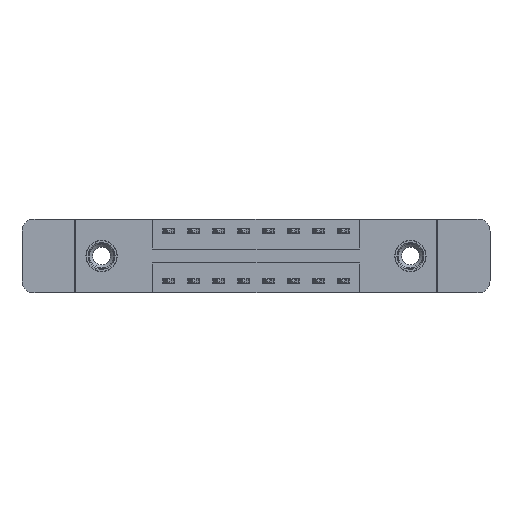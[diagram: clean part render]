
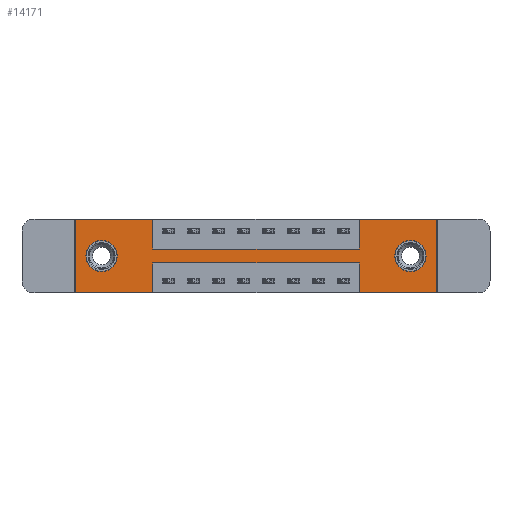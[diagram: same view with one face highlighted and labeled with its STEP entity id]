
A CAD part, front view. The second image highlights one B-rep face of the part: STEP entity #14171.
In plain terms, the highlighted planar face has unit normal (0, -1, 0).
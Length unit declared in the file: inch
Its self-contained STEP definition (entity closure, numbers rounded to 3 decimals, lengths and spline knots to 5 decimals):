
#9 = CARTESIAN_POINT ( 'NONE',  ( 1.6775, 0., -0.185 ) ) ;
#105 = ORIENTED_EDGE ( 'NONE', *, *, #8031, .F. ) ;
#212 = VECTOR ( 'NONE', #14831, 39.37008 ) ;
#493 = VERTEX_POINT ( 'NONE', #2565 ) ;
#850 = CIRCLE ( 'NONE', #13565, 0.078 ) ;
#884 = CARTESIAN_POINT ( 'NONE',  ( 0., 0., -0.37 ) ) ;
#892 = DIRECTION ( 'NONE',  ( 0., 0., -1. ) ) ;
#1053 = DIRECTION ( 'NONE',  ( 0., 0., -1. ) ) ;
#1204 = LINE ( 'NONE', #8077, #2448 ) ;
#1249 = VERTEX_POINT ( 'NONE', #8143 ) ;
#1659 = CIRCLE ( 'NONE', #5399, 0.078 ) ;
#1745 = CARTESIAN_POINT ( 'NONE',  ( 1.6775, 0., -0.185 ) ) ;
#1794 = DIRECTION ( 'NONE',  ( 0., 0., 1. ) ) ;
#1838 = EDGE_CURVE ( 'NONE', #9405, #1249, #10299, .T. ) ;
#1860 = DIRECTION ( 'NONE',  ( 0., 1., 0. ) ) ;
#1910 = DIRECTION ( 'NONE',  ( 0., 0., -1. ) ) ;
#1924 = CARTESIAN_POINT ( 'NONE',  ( 0., 0., -0.37 ) ) ;
#2002 = EDGE_CURVE ( 'NONE', #15263, #4245, #850, .T. ) ;
#2095 = CARTESIAN_POINT ( 'NONE',  ( 0.3875, 0., -0.22 ) ) ;
#2115 = EDGE_CURVE ( 'NONE', #8265, #6887, #10602, .T. ) ;
#2167 = EDGE_CURVE ( 'NONE', #6887, #2943, #5915, .T. ) ;
#2219 = EDGE_CURVE ( 'NONE', #12027, #9405, #13260, .T. ) ;
#2325 = ORIENTED_EDGE ( 'NONE', *, *, #8556, .F. ) ;
#2326 = DIRECTION ( 'NONE',  ( 0., 0., -1. ) ) ;
#2348 = ORIENTED_EDGE ( 'NONE', *, *, #10977, .F. ) ;
#2448 = VECTOR ( 'NONE', #13074, 39.37008 ) ;
#2565 = CARTESIAN_POINT ( 'NONE',  ( 1.81, 0., 0. ) ) ;
#2687 = LINE ( 'NONE', #14337, #8946 ) ;
#2885 = EDGE_LOOP ( 'NONE', ( #11225, #3592 ) ) ;
#2943 = VERTEX_POINT ( 'NONE', #4405 ) ;
#3103 = CARTESIAN_POINT ( 'NONE',  ( 1.4225, 0., 0. ) ) ;
#3215 = ORIENTED_EDGE ( 'NONE', *, *, #14825, .F. ) ;
#3223 = PLANE ( 'NONE',  #6197 ) ;
#3311 = VECTOR ( 'NONE', #1794, 39.37008 ) ;
#3425 = ORIENTED_EDGE ( 'NONE', *, *, #1838, .F. ) ;
#3592 = ORIENTED_EDGE ( 'NONE', *, *, #7766, .T. ) ;
#3636 = DIRECTION ( 'NONE',  ( 0., 0., 1. ) ) ;
#3756 = VERTEX_POINT ( 'NONE', #4872 ) ;
#3757 = ORIENTED_EDGE ( 'NONE', *, *, #9633, .F. ) ;
#3869 = CARTESIAN_POINT ( 'NONE',  ( 0.3875, 0., 0. ) ) ;
#4245 = VERTEX_POINT ( 'NONE', #10963 ) ;
#4341 = CARTESIAN_POINT ( 'NONE',  ( 0.3875, 0., -0.15 ) ) ;
#4405 = CARTESIAN_POINT ( 'NONE',  ( 0.3875, 0., -0.22 ) ) ;
#4727 = DIRECTION ( 'NONE',  ( 1., 0., 0. ) ) ;
#4756 = DIRECTION ( 'NONE',  ( 0., 1., 0. ) ) ;
#4807 = VECTOR ( 'NONE', #13497, 39.37008 ) ;
#4872 = CARTESIAN_POINT ( 'NONE',  ( 1.81, 0., -0.37 ) ) ;
#4967 = CARTESIAN_POINT ( 'NONE',  ( 0.1325, 0., -0.185 ) ) ;
#5260 = DIRECTION ( 'NONE',  ( 0., 0., -1. ) ) ;
#5300 = LINE ( 'NONE', #10060, #212 ) ;
#5338 = CARTESIAN_POINT ( 'NONE',  ( 0., 0., -0.37 ) ) ;
#5340 = VECTOR ( 'NONE', #3636, 39.37008 ) ;
#5399 = AXIS2_PLACEMENT_3D ( 'NONE', #4967, #12008, #7393 ) ;
#5503 = ORIENTED_EDGE ( 'NONE', *, *, #10831, .F. ) ;
#5666 = LINE ( 'NONE', #12925, #8121 ) ;
#5884 = AXIS2_PLACEMENT_3D ( 'NONE', #1745, #13371, #5260 ) ;
#5915 = LINE ( 'NONE', #2095, #7087 ) ;
#6039 = EDGE_CURVE ( 'NONE', #8719, #9441, #14628, .T. ) ;
#6043 = CARTESIAN_POINT ( 'NONE',  ( 1.6775, 0., -0.263 ) ) ;
#6099 = EDGE_LOOP ( 'NONE', ( #9477, #8108 ) ) ;
#6107 = ORIENTED_EDGE ( 'NONE', *, *, #2167, .F. ) ;
#6197 = AXIS2_PLACEMENT_3D ( 'NONE', #8146, #6667, #892 ) ;
#6465 = DIRECTION ( 'NONE',  ( -1., 0., 0. ) ) ;
#6659 = CARTESIAN_POINT ( 'NONE',  ( 1.6775, 0., -0.107 ) ) ;
#6667 = DIRECTION ( 'NONE',  ( 0., -1., 0. ) ) ;
#6802 = VERTEX_POINT ( 'NONE', #3869 ) ;
#6887 = VERTEX_POINT ( 'NONE', #10922 ) ;
#7087 = VECTOR ( 'NONE', #9290, 39.37008 ) ;
#7271 = CARTESIAN_POINT ( 'NONE',  ( 0., 0., 0. ) ) ;
#7393 = DIRECTION ( 'NONE',  ( 0., 0., 1. ) ) ;
#7656 = VERTEX_POINT ( 'NONE', #9230 ) ;
#7681 = ORIENTED_EDGE ( 'NONE', *, *, #13968, .F. ) ;
#7714 = VECTOR ( 'NONE', #6465, 39.37008 ) ;
#7766 = EDGE_CURVE ( 'NONE', #9441, #8719, #8418, .T. ) ;
#7866 = VECTOR ( 'NONE', #1910, 39.37008 ) ;
#8031 = EDGE_CURVE ( 'NONE', #6802, #12027, #5300, .T. ) ;
#8077 = CARTESIAN_POINT ( 'NONE',  ( 0., 0., 0. ) ) ;
#8108 = ORIENTED_EDGE ( 'NONE', *, *, #2002, .T. ) ;
#8121 = VECTOR ( 'NONE', #1053, 39.37008 ) ;
#8143 = CARTESIAN_POINT ( 'NONE',  ( 1.4225, 0., 0. ) ) ;
#8146 = CARTESIAN_POINT ( 'NONE',  ( 0., 0., -0.37 ) ) ;
#8265 = VERTEX_POINT ( 'NONE', #13025 ) ;
#8413 = CARTESIAN_POINT ( 'NONE',  ( 0.3875, 0., -0.15 ) ) ;
#8418 = CIRCLE ( 'NONE', #10175, 0.078 ) ;
#8556 = EDGE_CURVE ( 'NONE', #8740, #7656, #1204, .T. ) ;
#8719 = VERTEX_POINT ( 'NONE', #6659 ) ;
#8740 = VERTEX_POINT ( 'NONE', #5338 ) ;
#8749 = LINE ( 'NONE', #7271, #13620 ) ;
#8881 = LINE ( 'NONE', #1924, #7714 ) ;
#8946 = VECTOR ( 'NONE', #4727, 39.37008 ) ;
#9100 = CARTESIAN_POINT ( 'NONE',  ( 0.3875, 0., -0.37 ) ) ;
#9230 = CARTESIAN_POINT ( 'NONE',  ( 0., 0., 0. ) ) ;
#9290 = DIRECTION ( 'NONE',  ( -1., 0., 0. ) ) ;
#9405 = VERTEX_POINT ( 'NONE', #14403 ) ;
#9441 = VERTEX_POINT ( 'NONE', #6043 ) ;
#9477 = ORIENTED_EDGE ( 'NONE', *, *, #11855, .T. ) ;
#9571 = CARTESIAN_POINT ( 'NONE',  ( 0.1325, 0., -0.263 ) ) ;
#9633 = EDGE_CURVE ( 'NONE', #3756, #8265, #11514, .T. ) ;
#9936 = ORIENTED_EDGE ( 'NONE', *, *, #11493, .F. ) ;
#10060 = CARTESIAN_POINT ( 'NONE',  ( 0.3875, 0., 0. ) ) ;
#10072 = CARTESIAN_POINT ( 'NONE',  ( 0.1325, 0., -0.185 ) ) ;
#10175 = AXIS2_PLACEMENT_3D ( 'NONE', #9, #4756, #2326 ) ;
#10229 = DIRECTION ( 'NONE',  ( 0., 0., 1. ) ) ;
#10299 = LINE ( 'NONE', #3103, #3311 ) ;
#10569 = FACE_BOUND ( 'NONE', #6099, .T. ) ;
#10602 = LINE ( 'NONE', #13102, #5340 ) ;
#10831 = EDGE_CURVE ( 'NONE', #493, #3756, #13796, .T. ) ;
#10922 = CARTESIAN_POINT ( 'NONE',  ( 1.4225, 0., -0.22 ) ) ;
#10963 = CARTESIAN_POINT ( 'NONE',  ( 0.1325, 0., -0.107 ) ) ;
#10977 = EDGE_CURVE ( 'NONE', #2943, #12596, #5666, .T. ) ;
#11225 = ORIENTED_EDGE ( 'NONE', *, *, #6039, .T. ) ;
#11432 = DIRECTION ( 'NONE',  ( -1., 0., 0. ) ) ;
#11493 = EDGE_CURVE ( 'NONE', #7656, #6802, #8749, .T. ) ;
#11514 = LINE ( 'NONE', #884, #15129 ) ;
#11855 = EDGE_CURVE ( 'NONE', #4245, #15263, #1659, .T. ) ;
#12008 = DIRECTION ( 'NONE',  ( 0., 1., 0. ) ) ;
#12027 = VERTEX_POINT ( 'NONE', #4341 ) ;
#12280 = EDGE_LOOP ( 'NONE', ( #2348, #6107, #14221, #3757, #5503, #7681, #3425, #13765, #105, #9936, #2325, #3215 ) ) ;
#12596 = VERTEX_POINT ( 'NONE', #9100 ) ;
#12620 = CARTESIAN_POINT ( 'NONE',  ( 1.81, 0., 0. ) ) ;
#12925 = CARTESIAN_POINT ( 'NONE',  ( 0.3875, 0., -0.37 ) ) ;
#13025 = CARTESIAN_POINT ( 'NONE',  ( 1.4225, 0., -0.37 ) ) ;
#13074 = DIRECTION ( 'NONE',  ( 0., 0., 1. ) ) ;
#13102 = CARTESIAN_POINT ( 'NONE',  ( 1.4225, 0., -0.37 ) ) ;
#13260 = LINE ( 'NONE', #8413, #4807 ) ;
#13371 = DIRECTION ( 'NONE',  ( 0., 1., 0. ) ) ;
#13497 = DIRECTION ( 'NONE',  ( 1., 0., 0. ) ) ;
#13509 = DIRECTION ( 'NONE',  ( 1., 0., 0. ) ) ;
#13565 = AXIS2_PLACEMENT_3D ( 'NONE', #10072, #1860, #10229 ) ;
#13620 = VECTOR ( 'NONE', #13509, 39.37008 ) ;
#13765 = ORIENTED_EDGE ( 'NONE', *, *, #2219, .F. ) ;
#13796 = LINE ( 'NONE', #12620, #7866 ) ;
#13852 = FACE_OUTER_BOUND ( 'NONE', #12280, .T. ) ;
#13936 = FACE_BOUND ( 'NONE', #2885, .T. ) ;
#13968 = EDGE_CURVE ( 'NONE', #1249, #493, #2687, .T. ) ;
#14171 = ADVANCED_FACE ( 'NONE', ( #13936, #10569, #13852 ), #3223, .T. ) ;
#14221 = ORIENTED_EDGE ( 'NONE', *, *, #2115, .F. ) ;
#14337 = CARTESIAN_POINT ( 'NONE',  ( 0., 0., 0. ) ) ;
#14403 = CARTESIAN_POINT ( 'NONE',  ( 1.4225, 0., -0.15 ) ) ;
#14628 = CIRCLE ( 'NONE', #5884, 0.078 ) ;
#14825 = EDGE_CURVE ( 'NONE', #12596, #8740, #8881, .T. ) ;
#14831 = DIRECTION ( 'NONE',  ( 0., 0., -1. ) ) ;
#15129 = VECTOR ( 'NONE', #11432, 39.37008 ) ;
#15263 = VERTEX_POINT ( 'NONE', #9571 ) ;
